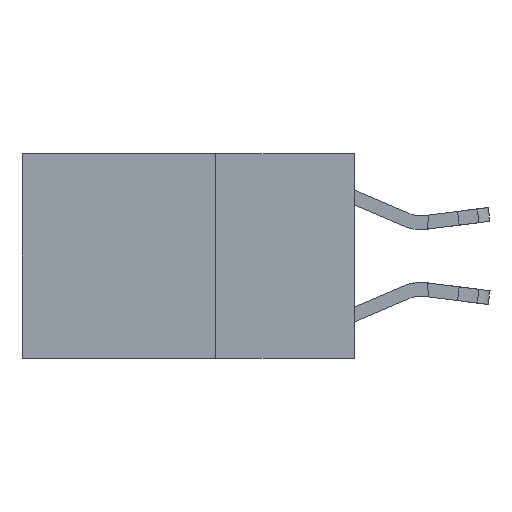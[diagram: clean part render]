
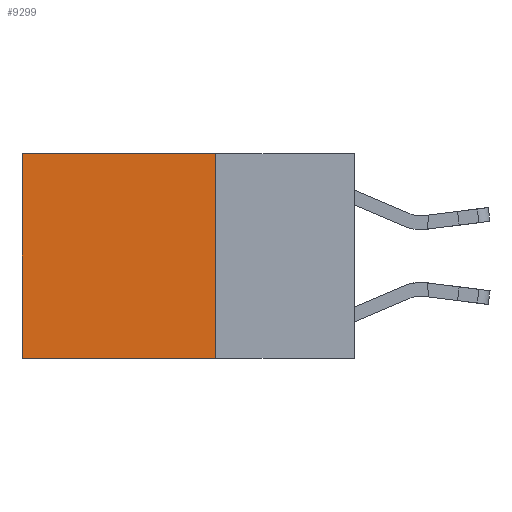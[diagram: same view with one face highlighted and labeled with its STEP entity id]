
A CAD part, left-side view. The second image highlights one B-rep face of the part: STEP entity #9299.
In plain terms, the highlighted planar face has unit normal (-1, 0, 0).
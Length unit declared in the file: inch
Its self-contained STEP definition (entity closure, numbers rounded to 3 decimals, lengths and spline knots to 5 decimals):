
#62 = CARTESIAN_POINT ( 'NONE',  ( 0.2625, 0.25, -0.37 ) ) ;
#243 = VECTOR ( 'NONE', #14991, 39.37008 ) ;
#314 = EDGE_CURVE ( 'NONE', #11354, #2509, #4543, .T. ) ;
#1353 = CARTESIAN_POINT ( 'NONE',  ( 0.2625, 0.6, -0.37 ) ) ;
#2389 = CARTESIAN_POINT ( 'NONE',  ( 0.2625, 0.6, 0. ) ) ;
#2509 = VERTEX_POINT ( 'NONE', #18425 ) ;
#3310 = AXIS2_PLACEMENT_3D ( 'NONE', #11857, #18242, #9065 ) ;
#4196 = VECTOR ( 'NONE', #4884, 39.37008 ) ;
#4486 = EDGE_CURVE ( 'NONE', #2509, #18104, #16205, .T. ) ;
#4543 = LINE ( 'NONE', #7431, #19261 ) ;
#4884 = DIRECTION ( 'NONE',  ( 0., 0., -1. ) ) ;
#6073 = LINE ( 'NONE', #9477, #4196 ) ;
#7187 = ORIENTED_EDGE ( 'NONE', *, *, #8068, .F. ) ;
#7211 = ORIENTED_EDGE ( 'NONE', *, *, #4486, .T. ) ;
#7431 = CARTESIAN_POINT ( 'NONE',  ( 0.2625, 0.25, 0. ) ) ;
#8068 = EDGE_CURVE ( 'NONE', #11354, #20029, #6073, .T. ) ;
#8861 = FACE_OUTER_BOUND ( 'NONE', #9748, .T. ) ;
#9065 = DIRECTION ( 'NONE',  ( 0., 0., -1. ) ) ;
#9299 = ADVANCED_FACE ( 'NONE', ( #8861 ), #10520, .F. ) ;
#9477 = CARTESIAN_POINT ( 'NONE',  ( 0.2625, 0.25, 0. ) ) ;
#9748 = EDGE_LOOP ( 'NONE', ( #7211, #19297, #7187, #14751 ) ) ;
#10233 = CARTESIAN_POINT ( 'NONE',  ( 0.2625, 0.25, 0. ) ) ;
#10336 = LINE ( 'NONE', #16623, #11552 ) ;
#10520 = PLANE ( 'NONE',  #3310 ) ;
#11354 = VERTEX_POINT ( 'NONE', #10233 ) ;
#11512 = EDGE_CURVE ( 'NONE', #20029, #18104, #10336, .T. ) ;
#11552 = VECTOR ( 'NONE', #15089, 39.37008 ) ;
#11857 = CARTESIAN_POINT ( 'NONE',  ( 0.2625, 0.25, 0. ) ) ;
#14751 = ORIENTED_EDGE ( 'NONE', *, *, #314, .T. ) ;
#14991 = DIRECTION ( 'NONE',  ( 0., 0., -1. ) ) ;
#15089 = DIRECTION ( 'NONE',  ( 0., 1., 0. ) ) ;
#16205 = LINE ( 'NONE', #2389, #243 ) ;
#16623 = CARTESIAN_POINT ( 'NONE',  ( 0.2625, 0.25, -0.37 ) ) ;
#16826 = DIRECTION ( 'NONE',  ( 0., 1., 0. ) ) ;
#18104 = VERTEX_POINT ( 'NONE', #1353 ) ;
#18242 = DIRECTION ( 'NONE',  ( 1., 0., 0. ) ) ;
#18425 = CARTESIAN_POINT ( 'NONE',  ( 0.2625, 0.6, 0. ) ) ;
#19261 = VECTOR ( 'NONE', #16826, 39.37008 ) ;
#19297 = ORIENTED_EDGE ( 'NONE', *, *, #11512, .F. ) ;
#20029 = VERTEX_POINT ( 'NONE', #62 ) ;
